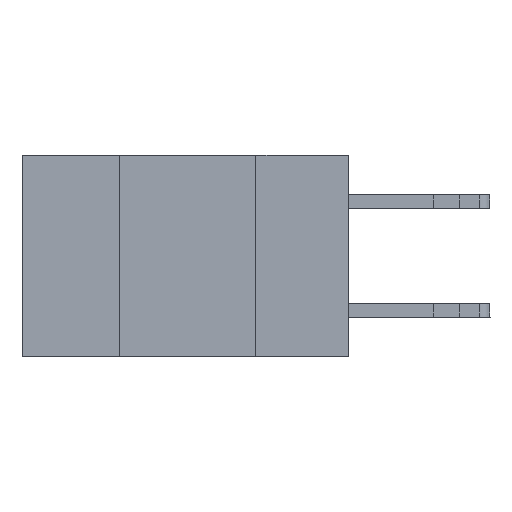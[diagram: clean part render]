
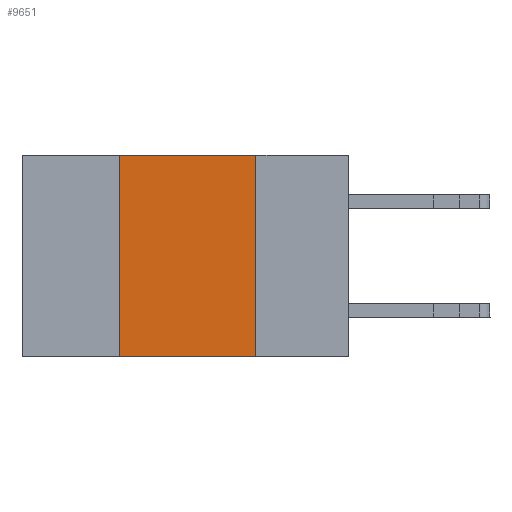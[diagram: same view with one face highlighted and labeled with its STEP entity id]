
A CAD part, left-side view. The second image highlights one B-rep face of the part: STEP entity #9651.
In plain terms, the highlighted planar face has unit normal (-1, 0, 0).
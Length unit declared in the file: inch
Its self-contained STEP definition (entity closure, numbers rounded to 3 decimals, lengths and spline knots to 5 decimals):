
#1213 = CARTESIAN_POINT ( 'NONE',  ( 0., 0.6, 0. ) ) ;
#2859 = VECTOR ( 'NONE', #7576, 39.37008 ) ;
#3140 = DIRECTION ( 'NONE',  ( 0., 0., 1. ) ) ;
#3937 = LINE ( 'NONE', #1213, #15222 ) ;
#4596 = EDGE_CURVE ( 'NONE', #9679, #6422, #11314, .T. ) ;
#4915 = CARTESIAN_POINT ( 'NONE',  ( 0., 0.42, 0. ) ) ;
#5590 = LINE ( 'NONE', #10053, #2859 ) ;
#6422 = VERTEX_POINT ( 'NONE', #14791 ) ;
#7576 = DIRECTION ( 'NONE',  ( 0., -1., 0. ) ) ;
#7741 = LINE ( 'NONE', #15678, #9327 ) ;
#8468 = VERTEX_POINT ( 'NONE', #16045 ) ;
#9327 = VECTOR ( 'NONE', #3140, 39.37008 ) ;
#9651 = ADVANCED_FACE ( 'NONE', ( #14935 ), #15183, .F. ) ;
#9679 = VERTEX_POINT ( 'NONE', #13956 ) ;
#9873 = DIRECTION ( 'NONE',  ( 0., 0., -1. ) ) ;
#9984 = CARTESIAN_POINT ( 'NONE',  ( 0., 0.17, 0. ) ) ;
#10046 = DIRECTION ( 'NONE',  ( 0., -1., 0. ) ) ;
#10053 = CARTESIAN_POINT ( 'NONE',  ( 0., 0.6, -0.37 ) ) ;
#10084 = DIRECTION ( 'NONE',  ( 1., 0., 0. ) ) ;
#10280 = ORIENTED_EDGE ( 'NONE', *, *, #12009, .F. ) ;
#10490 = EDGE_CURVE ( 'NONE', #8468, #6422, #5590, .T. ) ;
#11314 = LINE ( 'NONE', #9984, #12703 ) ;
#11705 = VERTEX_POINT ( 'NONE', #4915 ) ;
#11783 = AXIS2_PLACEMENT_3D ( 'NONE', #12575, #10084, #13892 ) ;
#12009 = EDGE_CURVE ( 'NONE', #8468, #11705, #7741, .T. ) ;
#12575 = CARTESIAN_POINT ( 'NONE',  ( 0., 0.6, 0. ) ) ;
#12703 = VECTOR ( 'NONE', #9873, 39.37008 ) ;
#13096 = ORIENTED_EDGE ( 'NONE', *, *, #4596, .F. ) ;
#13429 = EDGE_CURVE ( 'NONE', #11705, #9679, #3937, .T. ) ;
#13892 = DIRECTION ( 'NONE',  ( 0., 0., -1. ) ) ;
#13956 = CARTESIAN_POINT ( 'NONE',  ( 0., 0.17, 0. ) ) ;
#14440 = ORIENTED_EDGE ( 'NONE', *, *, #10490, .T. ) ;
#14562 = EDGE_LOOP ( 'NONE', ( #13096, #15365, #10280, #14440 ) ) ;
#14791 = CARTESIAN_POINT ( 'NONE',  ( 0., 0.17, -0.37 ) ) ;
#14935 = FACE_OUTER_BOUND ( 'NONE', #14562, .T. ) ;
#15183 = PLANE ( 'NONE',  #11783 ) ;
#15222 = VECTOR ( 'NONE', #10046, 39.37008 ) ;
#15365 = ORIENTED_EDGE ( 'NONE', *, *, #13429, .F. ) ;
#15678 = CARTESIAN_POINT ( 'NONE',  ( 0., 0.42, 0. ) ) ;
#16045 = CARTESIAN_POINT ( 'NONE',  ( 0., 0.42, -0.37 ) ) ;
